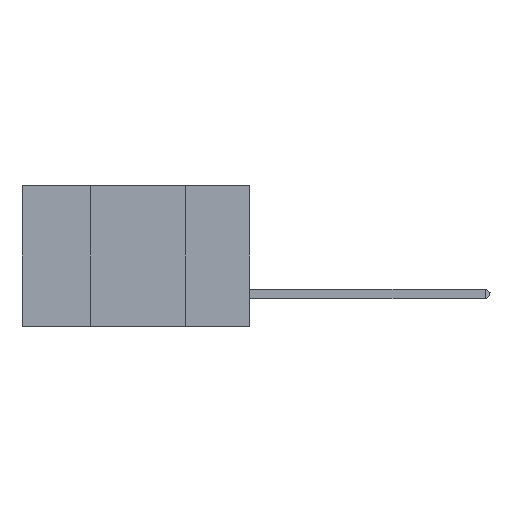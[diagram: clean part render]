
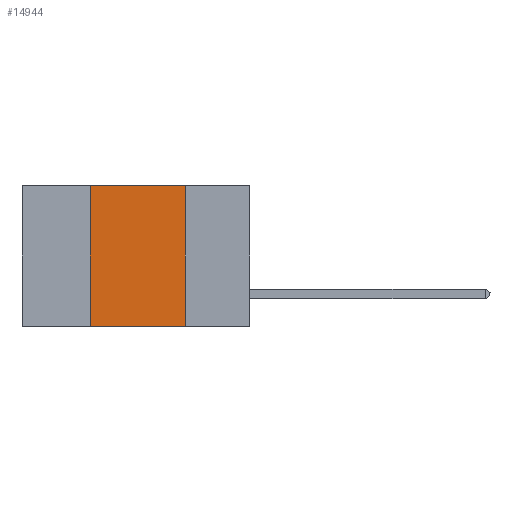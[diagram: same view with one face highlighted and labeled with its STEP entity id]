
A CAD part, left-side view. The second image highlights one B-rep face of the part: STEP entity #14944.
In plain terms, the highlighted planar face has unit normal (-1, 0, 0).
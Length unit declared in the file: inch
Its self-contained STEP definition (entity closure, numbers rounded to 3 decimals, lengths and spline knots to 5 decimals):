
#1271 = CARTESIAN_POINT ( 'NONE',  ( 0., 0.6, -0.37 ) ) ;
#1406 = VECTOR ( 'NONE', #15336, 39.37008 ) ;
#1897 = CARTESIAN_POINT ( 'NONE',  ( 0., 0.17, -0.37 ) ) ;
#2000 = VECTOR ( 'NONE', #37562, 39.37008 ) ;
#6239 = DIRECTION ( 'NONE',  ( 0., 0., -1. ) ) ;
#6919 = CARTESIAN_POINT ( 'NONE',  ( 0., 0.17, 0. ) ) ;
#9179 = LINE ( 'NONE', #33590, #11700 ) ;
#9194 = VECTOR ( 'NONE', #32070, 39.37008 ) ;
#9399 = EDGE_CURVE ( 'NONE', #29532, #35618, #33344, .T. ) ;
#9898 = PLANE ( 'NONE',  #38132 ) ;
#11700 = VECTOR ( 'NONE', #48606, 39.37008 ) ;
#12364 = ORIENTED_EDGE ( 'NONE', *, *, #42959, .T. ) ;
#13763 = DIRECTION ( 'NONE',  ( 1., 0., 0. ) ) ;
#14944 = ADVANCED_FACE ( 'NONE', ( #16291 ), #9898, .F. ) ;
#15336 = DIRECTION ( 'NONE',  ( 0., 0., 1. ) ) ;
#16291 = FACE_OUTER_BOUND ( 'NONE', #18553, .T. ) ;
#16902 = CARTESIAN_POINT ( 'NONE',  ( 0., 0.17, 0. ) ) ;
#18553 = EDGE_LOOP ( 'NONE', ( #32285, #34035, #44572, #12364 ) ) ;
#23951 = VERTEX_POINT ( 'NONE', #24793 ) ;
#24793 = CARTESIAN_POINT ( 'NONE',  ( 0., 0.42, 0. ) ) ;
#29532 = VERTEX_POINT ( 'NONE', #16902 ) ;
#29853 = LINE ( 'NONE', #45806, #1406 ) ;
#29954 = EDGE_CURVE ( 'NONE', #23951, #29532, #9179, .T. ) ;
#32070 = DIRECTION ( 'NONE',  ( 0., -1., 0. ) ) ;
#32285 = ORIENTED_EDGE ( 'NONE', *, *, #9399, .F. ) ;
#33051 = EDGE_CURVE ( 'NONE', #39815, #23951, #29853, .T. ) ;
#33344 = LINE ( 'NONE', #6919, #2000 ) ;
#33590 = CARTESIAN_POINT ( 'NONE',  ( 0., 0.6, 0. ) ) ;
#34035 = ORIENTED_EDGE ( 'NONE', *, *, #29954, .F. ) ;
#35618 = VERTEX_POINT ( 'NONE', #1897 ) ;
#37562 = DIRECTION ( 'NONE',  ( 0., 0., -1. ) ) ;
#38132 = AXIS2_PLACEMENT_3D ( 'NONE', #44756, #13763, #6239 ) ;
#39815 = VERTEX_POINT ( 'NONE', #47051 ) ;
#42959 = EDGE_CURVE ( 'NONE', #39815, #35618, #45869, .T. ) ;
#44572 = ORIENTED_EDGE ( 'NONE', *, *, #33051, .F. ) ;
#44756 = CARTESIAN_POINT ( 'NONE',  ( 0., 0.6, 0. ) ) ;
#45806 = CARTESIAN_POINT ( 'NONE',  ( 0., 0.42, 0. ) ) ;
#45869 = LINE ( 'NONE', #1271, #9194 ) ;
#47051 = CARTESIAN_POINT ( 'NONE',  ( 0., 0.42, -0.37 ) ) ;
#48606 = DIRECTION ( 'NONE',  ( 0., -1., 0. ) ) ;
